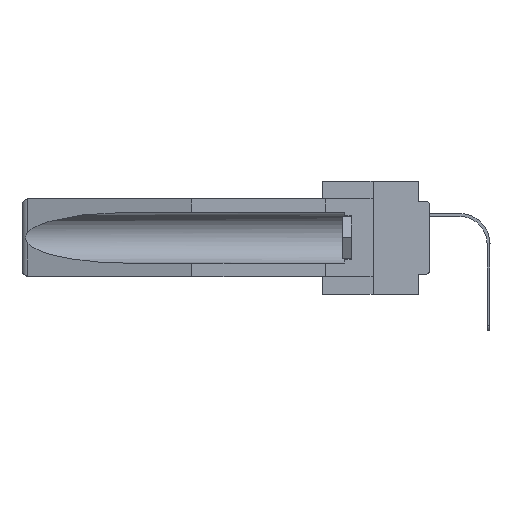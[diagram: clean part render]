
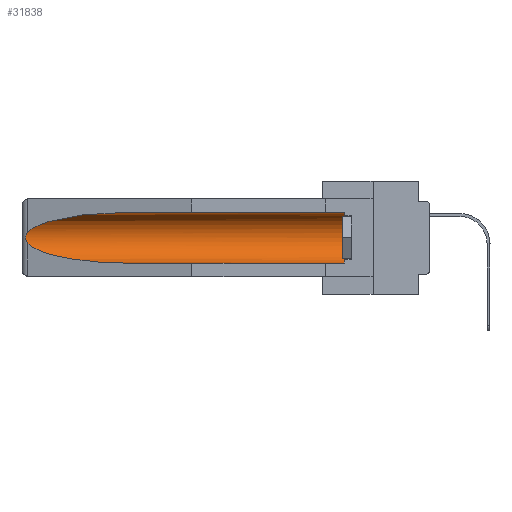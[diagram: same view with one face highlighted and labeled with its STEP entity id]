
A CAD part, left-side view. The second image highlights one B-rep face of the part: STEP entity #31838.
In plain terms, the highlighted cylindrical face has radius 2.857 mm (diameter 5.715 mm), a partial arc.
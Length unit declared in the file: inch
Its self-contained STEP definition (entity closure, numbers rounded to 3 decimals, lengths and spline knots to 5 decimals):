
#80 = ORIENTED_EDGE ( 'NONE', *, *, #25670, .T. ) ;
#1530 = CARTESIAN_POINT ( 'NONE',  ( 0.26537, 1.52718, -0.19328 ) ) ;
#1950 = VERTEX_POINT ( 'NONE', #9303 ) ;
#2251 = CARTESIAN_POINT ( 'NONE',  ( 0.155, 1.07973, -0.284 ) ) ;
#2480 = CARTESIAN_POINT ( 'NONE',  ( 0.155, -0.30754, -0.284 ) ) ;
#3537 = AXIS2_PLACEMENT_3D ( 'NONE', #4681, #23959, #34405 ) ;
#3566 = EDGE_CURVE ( 'NONE', #10153, #12449, #11255, .T. ) ;
#3686 = CARTESIAN_POINT ( 'NONE',  ( 0.155, 1.07973, -0.059 ) ) ;
#3809 = ORIENTED_EDGE ( 'NONE', *, *, #6811, .T. ) ;
#4084 = CARTESIAN_POINT ( 'NONE',  ( 0.25451, 1.48313, -0.24835 ) ) ;
#4261 = CARTESIAN_POINT ( 'NONE',  ( 0.155, 1.07973, -0.284 ) ) ;
#4681 = CARTESIAN_POINT ( 'NONE',  ( 0.155, -0.30754, -0.1715 ) ) ;
#6375 = B_SPLINE_CURVE_WITH_KNOTS ( 'NONE', 3,
 ( #29070, #34854, #29442, #15404, #10174, #20826, #26728, #13064, #16118, #31969 ),
 .UNSPECIFIED., .F., .F.,
 ( 4, 2, 2, 2, 4 ),
 ( 0., 0.00029, 0.00058, 0.00087, 0.00117 ),
 .UNSPECIFIED. ) ;
#6445 = CIRCLE ( 'NONE', #26600, 0.1125 ) ;
#6811 = EDGE_CURVE ( 'NONE', #12449, #22777, #32777, .T. ) ;
#7027 = ORIENTED_EDGE ( 'NONE', *, *, #12321, .T. ) ;
#7685 = VERTEX_POINT ( 'NONE', #2251 ) ;
#8021 = EDGE_LOOP ( 'NONE', ( #3809, #11858, #80, #16461, #7027, #21735 ) ) ;
#9099 =( BOUNDED_CURVE ( )  B_SPLINE_CURVE ( 3, ( #1530, #4084, #28928, #4261 ),
 .UNSPECIFIED., .F., .T. ) 
 B_SPLINE_CURVE_WITH_KNOTS ( ( 4, 4 ),
 ( 0.1948, 1.5708 ),
 .UNSPECIFIED. ) 
 CURVE ( )  GEOMETRIC_REPRESENTATION_ITEM ( )  RATIONAL_B_SPLINE_CURVE ( ( 1., 0.848, 0.848, 1. ) ) 
 REPRESENTATION_ITEM ( '' )  );
#9303 = CARTESIAN_POINT ( 'NONE',  ( 0.155, 0.126, -0.284 ) ) ;
#9455 = CARTESIAN_POINT ( 'NONE',  ( 0.25451, 1.48313, -0.09465 ) ) ;
#10153 = VERTEX_POINT ( 'NONE', #30123 ) ;
#10174 = CARTESIAN_POINT ( 'NONE',  ( 0.2675, 1.53308, -0.16763 ) ) ;
#10777 = DIRECTION ( 'NONE',  ( 0., 1., 0. ) ) ;
#11096 = CARTESIAN_POINT ( 'NONE',  ( 0.26537, 1.52718, -0.19328 ) ) ;
#11255 = LINE ( 'NONE', #22235, #15560 ) ;
#11858 = ORIENTED_EDGE ( 'NONE', *, *, #30918, .T. ) ;
#12321 = EDGE_CURVE ( 'NONE', #1950, #10153, #6445, .T. ) ;
#12449 = VERTEX_POINT ( 'NONE', #17313 ) ;
#13064 = CARTESIAN_POINT ( 'NONE',  ( 0.26655, 1.53094, -0.18657 ) ) ;
#13660 = LINE ( 'NONE', #2480, #18399 ) ;
#15404 = CARTESIAN_POINT ( 'NONE',  ( 0.2673, 1.5327, -0.16383 ) ) ;
#15429 = CARTESIAN_POINT ( 'NONE',  ( 0.26537, 1.52718, -0.14972 ) ) ;
#15560 = VECTOR ( 'NONE', #31053, 39.37008 ) ;
#16118 = CARTESIAN_POINT ( 'NONE',  ( 0.26597, 1.5296, -0.19026 ) ) ;
#16461 = ORIENTED_EDGE ( 'NONE', *, *, #23644, .F. ) ;
#17313 = CARTESIAN_POINT ( 'NONE',  ( 0.155, 1.07973, -0.059 ) ) ;
#18217 = FACE_OUTER_BOUND ( 'NONE', #8021, .T. ) ;
#18399 = VECTOR ( 'NONE', #10777, 39.37008 ) ;
#20826 = CARTESIAN_POINT ( 'NONE',  ( 0.2675, 1.53308, -0.17534 ) ) ;
#21484 = DIRECTION ( 'NONE',  ( 0., 0., 1. ) ) ;
#21735 = ORIENTED_EDGE ( 'NONE', *, *, #3566, .T. ) ;
#21810 = DIRECTION ( 'NONE',  ( 0., -1., 0. ) ) ;
#22235 = CARTESIAN_POINT ( 'NONE',  ( 0.155, -0.30754, -0.059 ) ) ;
#22777 = VERTEX_POINT ( 'NONE', #15429 ) ;
#23158 = CARTESIAN_POINT ( 'NONE',  ( 0.26537, 1.52718, -0.14972 ) ) ;
#23419 = CYLINDRICAL_SURFACE ( 'NONE', #3537, 0.1125 ) ;
#23644 = EDGE_CURVE ( 'NONE', #1950, #7685, #13660, .T. ) ;
#23959 = DIRECTION ( 'NONE',  ( 0., 1., 0. ) ) ;
#24349 = CARTESIAN_POINT ( 'NONE',  ( 0.155, 0.126, -0.1715 ) ) ;
#25299 = CARTESIAN_POINT ( 'NONE',  ( 0.21114, 1.30732, -0.059 ) ) ;
#25670 = EDGE_CURVE ( 'NONE', #34128, #7685, #9099, .T. ) ;
#26600 = AXIS2_PLACEMENT_3D ( 'NONE', #24349, #21810, #21484 ) ;
#26728 = CARTESIAN_POINT ( 'NONE',  ( 0.2673, 1.53269, -0.17917 ) ) ;
#28928 = CARTESIAN_POINT ( 'NONE',  ( 0.21114, 1.30732, -0.284 ) ) ;
#29070 = CARTESIAN_POINT ( 'NONE',  ( 0.26537, 1.52718, -0.14972 ) ) ;
#29442 = CARTESIAN_POINT ( 'NONE',  ( 0.26654, 1.53092, -0.15636 ) ) ;
#30123 = CARTESIAN_POINT ( 'NONE',  ( 0.155, 0.126, -0.059 ) ) ;
#30918 = EDGE_CURVE ( 'NONE', #22777, #34128, #6375, .T. ) ;
#31053 = DIRECTION ( 'NONE',  ( 0., 1., 0. ) ) ;
#31838 = ADVANCED_FACE ( 'NONE', ( #18217 ), #23419, .F. ) ;
#31969 = CARTESIAN_POINT ( 'NONE',  ( 0.26537, 1.52718, -0.19328 ) ) ;
#32777 =( BOUNDED_CURVE ( )  B_SPLINE_CURVE ( 3, ( #3686, #25299, #9455, #23158 ),
 .UNSPECIFIED., .F., .T. ) 
 B_SPLINE_CURVE_WITH_KNOTS ( ( 4, 4 ),
 ( 4.71239, 6.08839 ),
 .UNSPECIFIED. ) 
 CURVE ( )  GEOMETRIC_REPRESENTATION_ITEM ( )  RATIONAL_B_SPLINE_CURVE ( ( 1., 0.848, 0.848, 1. ) ) 
 REPRESENTATION_ITEM ( '' )  );
#34128 = VERTEX_POINT ( 'NONE', #11096 ) ;
#34405 = DIRECTION ( 'NONE',  ( 0., 0., 1. ) ) ;
#34854 = CARTESIAN_POINT ( 'NONE',  ( 0.26597, 1.52961, -0.15275 ) ) ;
